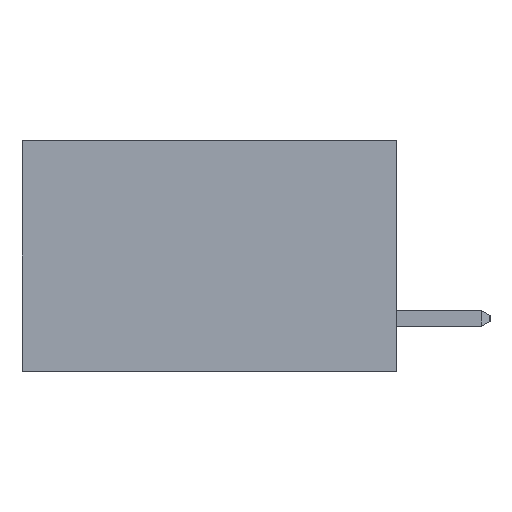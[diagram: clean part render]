
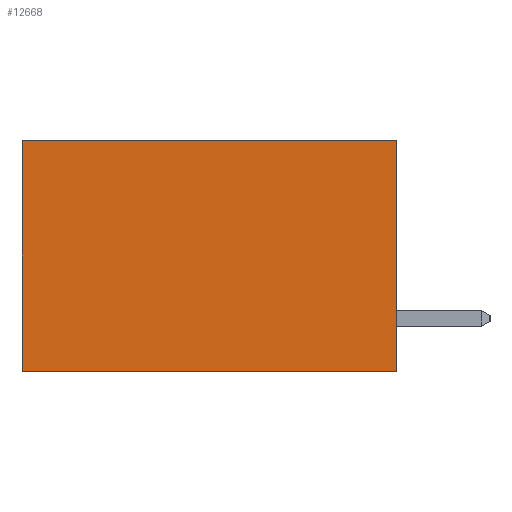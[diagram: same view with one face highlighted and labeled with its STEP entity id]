
A CAD part, left-side view. The second image highlights one B-rep face of the part: STEP entity #12668.
In plain terms, the highlighted planar face has unit normal (-1, 0, 0).
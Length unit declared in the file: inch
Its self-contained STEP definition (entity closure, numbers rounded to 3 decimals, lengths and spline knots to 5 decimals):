
#75 = ORIENTED_EDGE ( 'NONE', *, *, #10900, .F. ) ;
#1384 = PLANE ( 'NONE',  #22430 ) ;
#3276 = EDGE_CURVE ( 'NONE', #13951, #10084, #25928, .T. ) ;
#3782 = DIRECTION ( 'NONE',  ( 0., 0., -1. ) ) ;
#3908 = VECTOR ( 'NONE', #10098, 39.37008 ) ;
#5766 = DIRECTION ( 'NONE',  ( 0., 1., 0. ) ) ;
#8922 = VECTOR ( 'NONE', #10526, 39.37008 ) ;
#9282 = VERTEX_POINT ( 'NONE', #17844 ) ;
#10084 = VERTEX_POINT ( 'NONE', #27591 ) ;
#10098 = DIRECTION ( 'NONE',  ( 0., 0., -1. ) ) ;
#10305 = LINE ( 'NONE', #17074, #3908 ) ;
#10526 = DIRECTION ( 'NONE',  ( 0., 0., -1. ) ) ;
#10900 = EDGE_CURVE ( 'NONE', #18548, #13951, #10305, .T. ) ;
#12107 = ORIENTED_EDGE ( 'NONE', *, *, #29781, .T. ) ;
#12668 = ADVANCED_FACE ( 'NONE', ( #16444 ), #1384, .F. ) ;
#12741 = CARTESIAN_POINT ( 'NONE',  ( 0.298, 0., -0.37 ) ) ;
#12847 = DIRECTION ( 'NONE',  ( 0., 1., 0. ) ) ;
#13306 = CARTESIAN_POINT ( 'NONE',  ( 0.298, 0., 0. ) ) ;
#13951 = VERTEX_POINT ( 'NONE', #15810 ) ;
#15220 = LINE ( 'NONE', #29162, #8922 ) ;
#15810 = CARTESIAN_POINT ( 'NONE',  ( 0.298, 0., -0.37 ) ) ;
#16444 = FACE_OUTER_BOUND ( 'NONE', #25544, .T. ) ;
#16676 = ORIENTED_EDGE ( 'NONE', *, *, #22281, .T. ) ;
#17074 = CARTESIAN_POINT ( 'NONE',  ( 0.298, 0., 0. ) ) ;
#17844 = CARTESIAN_POINT ( 'NONE',  ( 0.298, 0.6, 0. ) ) ;
#17968 = DIRECTION ( 'NONE',  ( 1., 0., 0. ) ) ;
#18548 = VERTEX_POINT ( 'NONE', #30051 ) ;
#18794 = ORIENTED_EDGE ( 'NONE', *, *, #3276, .F. ) ;
#19698 = CARTESIAN_POINT ( 'NONE',  ( 0.298, 0., 0. ) ) ;
#19760 = VECTOR ( 'NONE', #5766, 39.37008 ) ;
#22281 = EDGE_CURVE ( 'NONE', #18548, #9282, #26107, .T. ) ;
#22430 = AXIS2_PLACEMENT_3D ( 'NONE', #13306, #17968, #3782 ) ;
#25544 = EDGE_LOOP ( 'NONE', ( #12107, #18794, #75, #16676 ) ) ;
#25928 = LINE ( 'NONE', #12741, #19760 ) ;
#26107 = LINE ( 'NONE', #19698, #30041 ) ;
#27591 = CARTESIAN_POINT ( 'NONE',  ( 0.298, 0.6, -0.37 ) ) ;
#29162 = CARTESIAN_POINT ( 'NONE',  ( 0.298, 0.6, 0. ) ) ;
#29781 = EDGE_CURVE ( 'NONE', #9282, #10084, #15220, .T. ) ;
#30041 = VECTOR ( 'NONE', #12847, 39.37008 ) ;
#30051 = CARTESIAN_POINT ( 'NONE',  ( 0.298, 0., 0. ) ) ;
